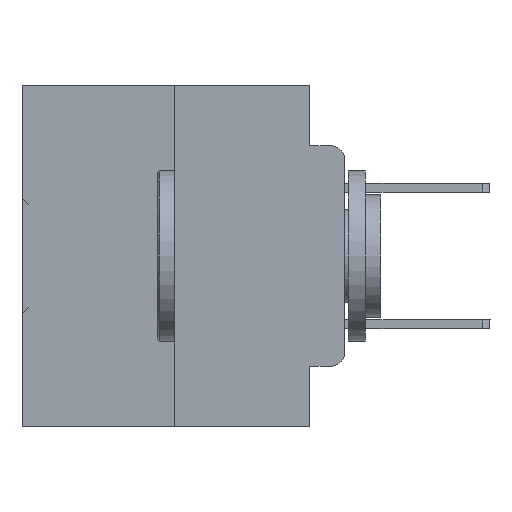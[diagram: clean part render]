
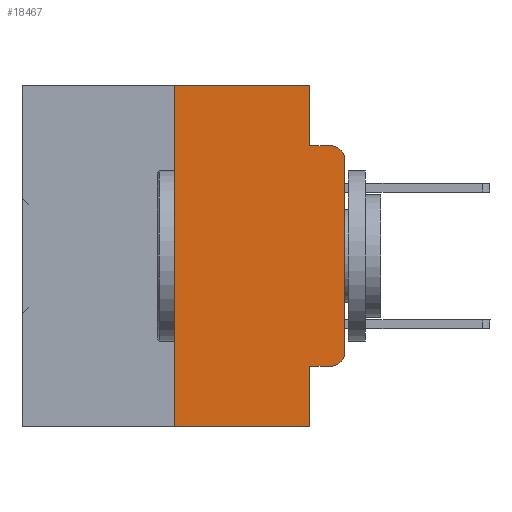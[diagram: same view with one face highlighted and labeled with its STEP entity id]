
A CAD part, left-side view. The second image highlights one B-rep face of the part: STEP entity #18467.
In plain terms, the highlighted planar face has unit normal (-1, 0, 0).
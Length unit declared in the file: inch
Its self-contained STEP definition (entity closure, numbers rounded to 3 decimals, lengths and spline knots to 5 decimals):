
#487 = EDGE_CURVE ( 'NONE', #31164, #23345, #20686, .T. ) ;
#556 = ORIENTED_EDGE ( 'NONE', *, *, #24400, .F. ) ;
#1062 = VERTEX_POINT ( 'NONE', #15527 ) ;
#2168 = DIRECTION ( 'NONE',  ( -1., 0., 0. ) ) ;
#2496 = AXIS2_PLACEMENT_3D ( 'NONE', #33488, #22396, #7925 ) ;
#2620 = DIRECTION ( 'NONE',  ( 0., 0., 1. ) ) ;
#3535 = EDGE_CURVE ( 'NONE', #10280, #24099, #35804, .T. ) ;
#3549 = VERTEX_POINT ( 'NONE', #4532 ) ;
#3566 = CARTESIAN_POINT ( 'NONE',  ( 0., 0.25, 0. ) ) ;
#3610 = EDGE_CURVE ( 'NONE', #23265, #9615, #31246, .T. ) ;
#4196 = EDGE_CURVE ( 'NONE', #10280, #9615, #10587, .T. ) ;
#4532 = CARTESIAN_POINT ( 'NONE',  ( 0., 0.051, -0.0885 ) ) ;
#5125 = PLANE ( 'NONE',  #28406 ) ;
#6101 = VECTOR ( 'NONE', #30063, 39.37008 ) ;
#6686 = EDGE_CURVE ( 'NONE', #1062, #20654, #17097, .T. ) ;
#7394 = DIRECTION ( 'NONE',  ( 0., -1., 0. ) ) ;
#7548 = CARTESIAN_POINT ( 'NONE',  ( 0., 0.051, 0. ) ) ;
#7729 = EDGE_CURVE ( 'NONE', #23345, #3549, #20011, .T. ) ;
#7925 = DIRECTION ( 'NONE',  ( 0., 0., -1. ) ) ;
#8080 = CARTESIAN_POINT ( 'NONE',  ( 0., 0., -0.1085 ) ) ;
#8387 = CARTESIAN_POINT ( 'NONE',  ( 0., 0.051, -0.5 ) ) ;
#8597 = DIRECTION ( 'NONE',  ( 0., 0., -1. ) ) ;
#8811 = CARTESIAN_POINT ( 'NONE',  ( 0., 0.051, -0.0885 ) ) ;
#9615 = VERTEX_POINT ( 'NONE', #8387 ) ;
#10280 = VERTEX_POINT ( 'NONE', #26367 ) ;
#10433 = VECTOR ( 'NONE', #8597, 39.37008 ) ;
#10467 = ORIENTED_EDGE ( 'NONE', *, *, #23910, .F. ) ;
#10587 = LINE ( 'NONE', #7548, #32165 ) ;
#10844 = DIRECTION ( 'NONE',  ( 1., 0., 0. ) ) ;
#11024 = DIRECTION ( 'NONE',  ( 0., 0., -1. ) ) ;
#12178 = CARTESIAN_POINT ( 'NONE',  ( 0., 0.02, -0.0885 ) ) ;
#13674 = CARTESIAN_POINT ( 'NONE',  ( 0., 0.051, 0. ) ) ;
#13862 = VERTEX_POINT ( 'NONE', #12178 ) ;
#14660 = VECTOR ( 'NONE', #2620, 39.37008 ) ;
#15527 = CARTESIAN_POINT ( 'NONE',  ( 0., 0., -0.3915 ) ) ;
#15848 = CIRCLE ( 'NONE', #2496, 0.02 ) ;
#17097 = LINE ( 'NONE', #19551, #14660 ) ;
#18328 = ORIENTED_EDGE ( 'NONE', *, *, #487, .F. ) ;
#18467 = ADVANCED_FACE ( 'NONE', ( #25699 ), #5125, .F. ) ;
#19158 = CARTESIAN_POINT ( 'NONE',  ( 0., 0.25, -0.5 ) ) ;
#19319 = ORIENTED_EDGE ( 'NONE', *, *, #6686, .T. ) ;
#19551 = CARTESIAN_POINT ( 'NONE',  ( 0., 0., 0. ) ) ;
#20011 = LINE ( 'NONE', #23248, #10433 ) ;
#20654 = VERTEX_POINT ( 'NONE', #8080 ) ;
#20686 = LINE ( 'NONE', #26798, #23797 ) ;
#20846 = ORIENTED_EDGE ( 'NONE', *, *, #7729, .F. ) ;
#21203 = ORIENTED_EDGE ( 'NONE', *, *, #22466, .T. ) ;
#22396 = DIRECTION ( 'NONE',  ( -1., 0., 0. ) ) ;
#22466 = EDGE_CURVE ( 'NONE', #20654, #13862, #25478, .T. ) ;
#23248 = CARTESIAN_POINT ( 'NONE',  ( 0., 0.051, 0. ) ) ;
#23265 = VERTEX_POINT ( 'NONE', #19158 ) ;
#23345 = VERTEX_POINT ( 'NONE', #13674 ) ;
#23797 = VECTOR ( 'NONE', #26995, 39.37008 ) ;
#23835 = DIRECTION ( 'NONE',  ( 0., -1., 0. ) ) ;
#23910 = EDGE_CURVE ( 'NONE', #3549, #13862, #27407, .T. ) ;
#24099 = VERTEX_POINT ( 'NONE', #25129 ) ;
#24400 = EDGE_CURVE ( 'NONE', #23265, #31164, #32735, .T. ) ;
#24465 = EDGE_CURVE ( 'NONE', #24099, #1062, #15848, .T. ) ;
#24614 = ORIENTED_EDGE ( 'NONE', *, *, #3535, .T. ) ;
#25129 = CARTESIAN_POINT ( 'NONE',  ( 0., 0.02, -0.4115 ) ) ;
#25478 = CIRCLE ( 'NONE', #36414, 0.02 ) ;
#25514 = CARTESIAN_POINT ( 'NONE',  ( 0., 0.473, 0. ) ) ;
#25699 = FACE_OUTER_BOUND ( 'NONE', #27599, .T. ) ;
#26367 = CARTESIAN_POINT ( 'NONE',  ( 0., 0.051, -0.4115 ) ) ;
#26798 = CARTESIAN_POINT ( 'NONE',  ( 0., 0.473, 0. ) ) ;
#26995 = DIRECTION ( 'NONE',  ( 0., -1., 0. ) ) ;
#27407 = LINE ( 'NONE', #8811, #35877 ) ;
#27599 = EDGE_LOOP ( 'NONE', ( #19319, #21203, #10467, #20846, #18328, #556, #37300, #36610, #24614, #29547 ) ) ;
#27948 = CARTESIAN_POINT ( 'NONE',  ( 0., 0.25, 0. ) ) ;
#28406 = AXIS2_PLACEMENT_3D ( 'NONE', #25514, #10844, #11024 ) ;
#28550 = CARTESIAN_POINT ( 'NONE',  ( 0., 0.473, -0.5 ) ) ;
#29547 = ORIENTED_EDGE ( 'NONE', *, *, #24465, .T. ) ;
#30063 = DIRECTION ( 'NONE',  ( 0., 0., 1. ) ) ;
#30547 = CARTESIAN_POINT ( 'NONE',  ( 0., 0.02, -0.1085 ) ) ;
#30704 = VECTOR ( 'NONE', #7394, 39.37008 ) ;
#30815 = DIRECTION ( 'NONE',  ( 0., 0., -1. ) ) ;
#31164 = VERTEX_POINT ( 'NONE', #27948 ) ;
#31246 = LINE ( 'NONE', #28550, #31559 ) ;
#31559 = VECTOR ( 'NONE', #33918, 39.37008 ) ;
#32165 = VECTOR ( 'NONE', #30815, 39.37008 ) ;
#32735 = LINE ( 'NONE', #3566, #6101 ) ;
#33488 = CARTESIAN_POINT ( 'NONE',  ( 0., 0.02, -0.3915 ) ) ;
#33519 = CARTESIAN_POINT ( 'NONE',  ( 0., 0.051, -0.4115 ) ) ;
#33918 = DIRECTION ( 'NONE',  ( 0., -1., 0. ) ) ;
#35804 = LINE ( 'NONE', #33519, #30704 ) ;
#35877 = VECTOR ( 'NONE', #23835, 39.37008 ) ;
#36414 = AXIS2_PLACEMENT_3D ( 'NONE', #30547, #2168, #36446 ) ;
#36446 = DIRECTION ( 'NONE',  ( 0., 0., -1. ) ) ;
#36610 = ORIENTED_EDGE ( 'NONE', *, *, #4196, .F. ) ;
#37300 = ORIENTED_EDGE ( 'NONE', *, *, #3610, .T. ) ;
